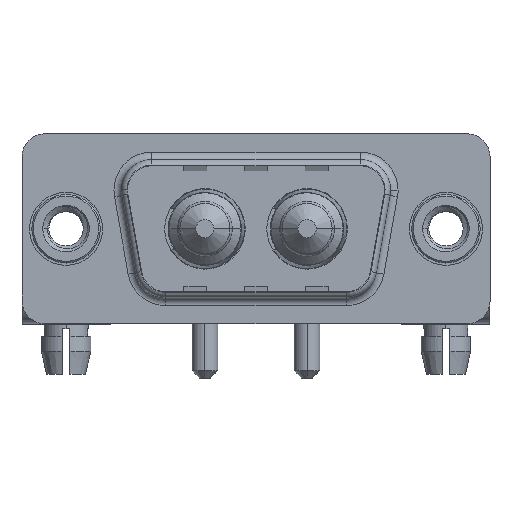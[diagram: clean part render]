
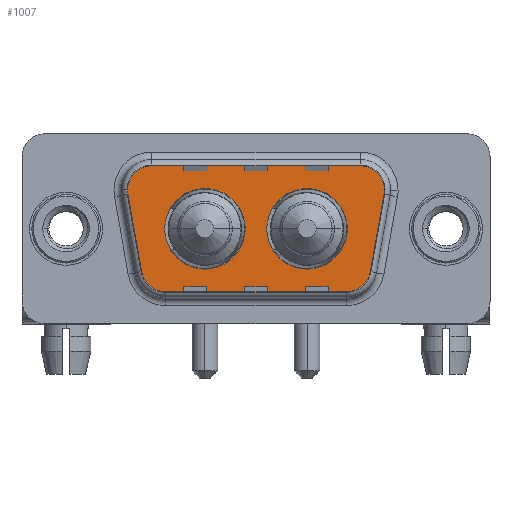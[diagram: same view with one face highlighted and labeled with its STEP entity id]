
A CAD part, top view. The second image highlights one B-rep face of the part: STEP entity #1007.
In plain terms, the highlighted planar face has unit normal (0, 0, 1).
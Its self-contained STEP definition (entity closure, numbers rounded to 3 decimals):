
#33 = CIRCLE ( 'NONE', #1992, 2. ) ;
#301 = CARTESIAN_POINT ( 'NONE',  ( 9.14, 0., 0. ) ) ;
#506 = VERTEX_POINT ( 'NONE', #6265 ) ;
#596 = DIRECTION ( 'NONE',  ( -1., 0., 0. ) ) ;
#641 = ORIENTED_EDGE ( 'NONE', *, *, #2474, .T. ) ;
#650 = CARTESIAN_POINT ( 'NONE',  ( 20.511, -3.247, 0. ) ) ;
#755 = AXIS2_PLACEMENT_3D ( 'NONE', #1330, #8320, #10400 ) ;
#1007 = ADVANCED_FACE ( 'NONE', ( #13345, #8531, #2895 ), #2674, .T. ) ;
#1013 = ORIENTED_EDGE ( 'NONE', *, *, #11425, .T. ) ;
#1172 = DIRECTION ( 'NONE',  ( 0.174, 0.985, 0. ) ) ;
#1207 = VERTEX_POINT ( 'NONE', #5782 ) ;
#1212 = CARTESIAN_POINT ( 'NONE',  ( 5.436, 4.9, 0. ) ) ;
#1330 = CARTESIAN_POINT ( 'NONE',  ( 6.459, -2.9, 0. ) ) ;
#1511 = CIRCLE ( 'NONE', #5889, 2. ) ;
#1642 = ORIENTED_EDGE ( 'NONE', *, *, #4388, .F. ) ;
#1740 = AXIS2_PLACEMENT_3D ( 'NONE', #301, #8370, #7162 ) ;
#1817 = DIRECTION ( 'NONE',  ( 0., 0., 1. ) ) ;
#1992 = AXIS2_PLACEMENT_3D ( 'NONE', #3862, #3937, #7356 ) ;
#2200 = EDGE_LOOP ( 'NONE', ( #10723, #13255 ) ) ;
#2474 = EDGE_CURVE ( 'NONE', #3222, #5968, #14895, .T. ) ;
#2579 = EDGE_CURVE ( 'NONE', #5987, #1207, #14669, .T. ) ;
#2674 = PLANE ( 'NONE',  #8674 ) ;
#2740 = VECTOR ( 'NONE', #9739, 1000. ) ;
#2771 = CARTESIAN_POINT ( 'NONE',  ( 15.86, 0., 0. ) ) ;
#2782 = VECTOR ( 'NONE', #596, 1000. ) ;
#2895 = FACE_OUTER_BOUND ( 'NONE', #6167, .T. ) ;
#2910 = CARTESIAN_POINT ( 'NONE',  ( 19.564, 4.9, 0. ) ) ;
#3026 = DIRECTION ( 'NONE',  ( 0., 0., 1. ) ) ;
#3116 = CARTESIAN_POINT ( 'NONE',  ( 5.436, 2.9, 0. ) ) ;
#3222 = VERTEX_POINT ( 'NONE', #5328 ) ;
#3374 = VERTEX_POINT ( 'NONE', #1212 ) ;
#3513 = VECTOR ( 'NONE', #4191, 1000. ) ;
#3862 = CARTESIAN_POINT ( 'NONE',  ( 19.564, 2.9, 0. ) ) ;
#3921 = CIRCLE ( 'NONE', #1740, 2.65 ) ;
#3937 = DIRECTION ( 'NONE',  ( 0., 0., 1. ) ) ;
#3955 = CARTESIAN_POINT ( 'NONE',  ( 3.466, 2.553, 0. ) ) ;
#4070 = ORIENTED_EDGE ( 'NONE', *, *, #9239, .T. ) ;
#4188 = CIRCLE ( 'NONE', #6129, 2.65 ) ;
#4191 = DIRECTION ( 'NONE',  ( 1., 0., 0. ) ) ;
#4388 = EDGE_CURVE ( 'NONE', #1207, #5987, #4188, .T. ) ;
#4511 = ORIENTED_EDGE ( 'NONE', *, *, #13228, .T. ) ;
#4970 = DIRECTION ( 'NONE',  ( 0., 0., 1. ) ) ;
#5248 = DIRECTION ( 'NONE',  ( 0., 0., 1. ) ) ;
#5328 = CARTESIAN_POINT ( 'NONE',  ( 4.489, -3.247, 0. ) ) ;
#5426 = CARTESIAN_POINT ( 'NONE',  ( 11.79, 0., 0. ) ) ;
#5533 = VERTEX_POINT ( 'NONE', #7890 ) ;
#5658 = AXIS2_PLACEMENT_3D ( 'NONE', #3116, #1817, #11187 ) ;
#5782 = CARTESIAN_POINT ( 'NONE',  ( 18.51, 0., 0. ) ) ;
#5860 = CIRCLE ( 'NONE', #12682, 2. ) ;
#5889 = AXIS2_PLACEMENT_3D ( 'NONE', #14616, #3026, #6681 ) ;
#5968 = VERTEX_POINT ( 'NONE', #11078 ) ;
#5987 = VERTEX_POINT ( 'NONE', #7789 ) ;
#6129 = AXIS2_PLACEMENT_3D ( 'NONE', #9583, #14262, #8442 ) ;
#6155 = DIRECTION ( 'NONE',  ( 1., 0., 0. ) ) ;
#6167 = EDGE_LOOP ( 'NONE', ( #10361, #13233, #12012, #4070, #4511, #11935, #13239, #641, #1013 ) ) ;
#6265 = CARTESIAN_POINT ( 'NONE',  ( 6.49, 0., 0. ) ) ;
#6346 = DIRECTION ( 'NONE',  ( 1., 0., 0. ) ) ;
#6443 = VERTEX_POINT ( 'NONE', #2910 ) ;
#6681 = DIRECTION ( 'NONE',  ( 1., 0., 0. ) ) ;
#6767 = LINE ( 'NONE', #13557, #2782 ) ;
#7162 = DIRECTION ( 'NONE',  ( 1., 0., 0. ) ) ;
#7310 = DIRECTION ( 'NONE',  ( 1., 0., 0. ) ) ;
#7341 = AXIS2_PLACEMENT_3D ( 'NONE', #2771, #4970, #6346 ) ;
#7356 = DIRECTION ( 'NONE',  ( -1., 0., 0. ) ) ;
#7511 = VERTEX_POINT ( 'NONE', #13791 ) ;
#7789 = CARTESIAN_POINT ( 'NONE',  ( 13.21, 0., 0. ) ) ;
#7843 = CARTESIAN_POINT ( 'NONE',  ( 6.459, -4.9, 0. ) ) ;
#7890 = CARTESIAN_POINT ( 'NONE',  ( 3.466, 2.553, 0. ) ) ;
#7895 = VERTEX_POINT ( 'NONE', #5426 ) ;
#8162 = CARTESIAN_POINT ( 'NONE',  ( 18.541, -4.9, 0. ) ) ;
#8172 = VERTEX_POINT ( 'NONE', #8162 ) ;
#8192 = EDGE_CURVE ( 'NONE', #14911, #7511, #5860, .T. ) ;
#8320 = DIRECTION ( 'NONE',  ( 0., 0., 1. ) ) ;
#8370 = DIRECTION ( 'NONE',  ( 0., 0., 1. ) ) ;
#8442 = DIRECTION ( 'NONE',  ( 1., 0., 0. ) ) ;
#8531 = FACE_BOUND ( 'NONE', #2200, .T. ) ;
#8597 = LINE ( 'NONE', #3955, #2740 ) ;
#8604 = CARTESIAN_POINT ( 'NONE',  ( 18.541, -2.9, 0. ) ) ;
#8668 = CARTESIAN_POINT ( 'NONE',  ( 21.534, 2.553, 0. ) ) ;
#8674 = AXIS2_PLACEMENT_3D ( 'NONE', #8604, #5248, #7310 ) ;
#8686 = EDGE_CURVE ( 'NONE', #7895, #506, #3921, .T. ) ;
#9239 = EDGE_CURVE ( 'NONE', #7511, #6443, #33, .T. ) ;
#9406 = EDGE_CURVE ( 'NONE', #8172, #13705, #1511, .T. ) ;
#9579 = DIRECTION ( 'NONE',  ( 0., 0., 1. ) ) ;
#9583 = CARTESIAN_POINT ( 'NONE',  ( 15.86, 0., 0. ) ) ;
#9739 = DIRECTION ( 'NONE',  ( 0.174, -0.985, 0. ) ) ;
#10102 = EDGE_LOOP ( 'NONE', ( #1642, #14038 ) ) ;
#10185 = EDGE_CURVE ( 'NONE', #5533, #3222, #8597, .T. ) ;
#10361 = ORIENTED_EDGE ( 'NONE', *, *, #9406, .T. ) ;
#10400 = DIRECTION ( 'NONE',  ( -1., 0., 0. ) ) ;
#10536 = DIRECTION ( 'NONE',  ( 0., 0., 1. ) ) ;
#10558 = CIRCLE ( 'NONE', #13488, 2.65 ) ;
#10723 = ORIENTED_EDGE ( 'NONE', *, *, #8686, .F. ) ;
#11078 = CARTESIAN_POINT ( 'NONE',  ( 6.459, -4.9, 0. ) ) ;
#11187 = DIRECTION ( 'NONE',  ( 1., 0., 0. ) ) ;
#11425 = EDGE_CURVE ( 'NONE', #5968, #8172, #14882, .T. ) ;
#11645 = EDGE_CURVE ( 'NONE', #506, #7895, #10558, .T. ) ;
#11913 = EDGE_CURVE ( 'NONE', #3374, #5533, #13713, .T. ) ;
#11935 = ORIENTED_EDGE ( 'NONE', *, *, #11913, .T. ) ;
#12012 = ORIENTED_EDGE ( 'NONE', *, *, #8192, .T. ) ;
#12682 = AXIS2_PLACEMENT_3D ( 'NONE', #12986, #10536, #13064 ) ;
#12700 = CARTESIAN_POINT ( 'NONE',  ( 21.534, 2.553, 0. ) ) ;
#12986 = CARTESIAN_POINT ( 'NONE',  ( 19.564, 2.9, 0. ) ) ;
#13064 = DIRECTION ( 'NONE',  ( -1., 0., 0. ) ) ;
#13112 = CARTESIAN_POINT ( 'NONE',  ( 9.14, 0., 0. ) ) ;
#13228 = EDGE_CURVE ( 'NONE', #6443, #3374, #6767, .T. ) ;
#13233 = ORIENTED_EDGE ( 'NONE', *, *, #13892, .T. ) ;
#13239 = ORIENTED_EDGE ( 'NONE', *, *, #10185, .T. ) ;
#13255 = ORIENTED_EDGE ( 'NONE', *, *, #11645, .F. ) ;
#13345 = FACE_BOUND ( 'NONE', #10102, .T. ) ;
#13488 = AXIS2_PLACEMENT_3D ( 'NONE', #13112, #9579, #6155 ) ;
#13557 = CARTESIAN_POINT ( 'NONE',  ( 5.436, 4.9, 0. ) ) ;
#13705 = VERTEX_POINT ( 'NONE', #650 ) ;
#13713 = CIRCLE ( 'NONE', #5658, 2. ) ;
#13791 = CARTESIAN_POINT ( 'NONE',  ( 21.564, 2.9, 0. ) ) ;
#13892 = EDGE_CURVE ( 'NONE', #13705, #14911, #15072, .T. ) ;
#14038 = ORIENTED_EDGE ( 'NONE', *, *, #2579, .F. ) ;
#14262 = DIRECTION ( 'NONE',  ( 0., 0., 1. ) ) ;
#14616 = CARTESIAN_POINT ( 'NONE',  ( 18.541, -2.9, 0. ) ) ;
#14669 = CIRCLE ( 'NONE', #7341, 2.65 ) ;
#14882 = LINE ( 'NONE', #7843, #3513 ) ;
#14895 = CIRCLE ( 'NONE', #755, 2. ) ;
#14911 = VERTEX_POINT ( 'NONE', #8668 ) ;
#14985 = VECTOR ( 'NONE', #1172, 1000. ) ;
#15072 = LINE ( 'NONE', #12700, #14985 ) ;
